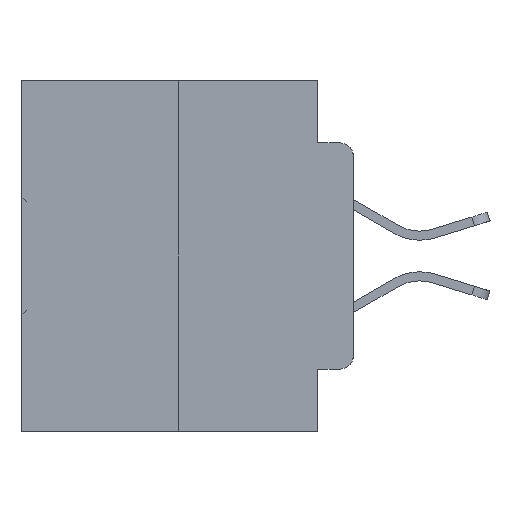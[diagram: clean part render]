
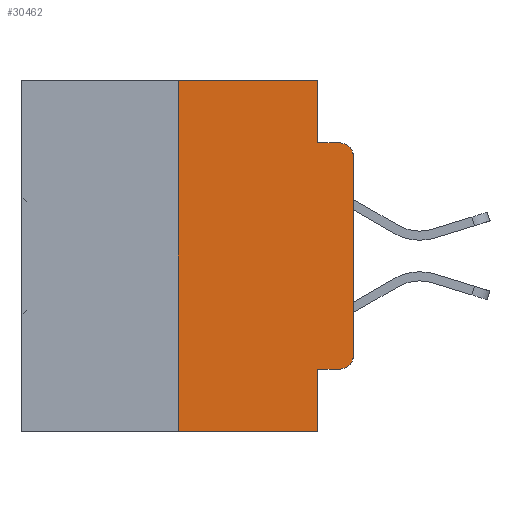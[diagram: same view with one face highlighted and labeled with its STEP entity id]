
A CAD part, left-side view. The second image highlights one B-rep face of the part: STEP entity #30462.
In plain terms, the highlighted planar face has unit normal (-1, 0, 0).
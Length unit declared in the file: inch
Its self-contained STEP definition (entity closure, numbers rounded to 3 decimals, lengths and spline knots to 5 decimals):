
#156 = VERTEX_POINT ( 'NONE', #30643 ) ;
#760 = CARTESIAN_POINT ( 'NONE',  ( 0., 0.02, -0.4115 ) ) ;
#1141 = LINE ( 'NONE', #17078, #32372 ) ;
#1329 = EDGE_CURVE ( 'NONE', #8451, #25424, #10565, .T. ) ;
#2308 = ORIENTED_EDGE ( 'NONE', *, *, #17597, .T. ) ;
#2309 = VERTEX_POINT ( 'NONE', #15167 ) ;
#2852 = LINE ( 'NONE', #10535, #20112 ) ;
#3931 = VERTEX_POINT ( 'NONE', #33849 ) ;
#4574 = EDGE_CURVE ( 'NONE', #19548, #156, #23249, .T. ) ;
#4688 = ORIENTED_EDGE ( 'NONE', *, *, #20201, .T. ) ;
#4934 = DIRECTION ( 'NONE',  ( -1., 0., 0. ) ) ;
#6073 = EDGE_CURVE ( 'NONE', #8706, #3931, #33449, .T. ) ;
#6129 = DIRECTION ( 'NONE',  ( 0., 0., -1. ) ) ;
#6868 = CARTESIAN_POINT ( 'NONE',  ( 0., 0.473, 0. ) ) ;
#7009 = VECTOR ( 'NONE', #31491, 39.37008 ) ;
#8111 = DIRECTION ( 'NONE',  ( 0., 0., 1. ) ) ;
#8451 = VERTEX_POINT ( 'NONE', #20115 ) ;
#8706 = VERTEX_POINT ( 'NONE', #21029 ) ;
#8824 = ORIENTED_EDGE ( 'NONE', *, *, #12725, .T. ) ;
#9120 = EDGE_CURVE ( 'NONE', #19548, #24279, #12750, .T. ) ;
#9899 = LINE ( 'NONE', #20765, #22254 ) ;
#9903 = ORIENTED_EDGE ( 'NONE', *, *, #17345, .F. ) ;
#10204 = CARTESIAN_POINT ( 'NONE',  ( 0., 0.02, -0.3915 ) ) ;
#10334 = CARTESIAN_POINT ( 'NONE',  ( 0., 0.051, -0.4115 ) ) ;
#10535 = CARTESIAN_POINT ( 'NONE',  ( 0., 0.051, -0.0885 ) ) ;
#10545 = LINE ( 'NONE', #23977, #12593 ) ;
#10565 = LINE ( 'NONE', #25010, #22072 ) ;
#11326 = EDGE_CURVE ( 'NONE', #15008, #2309, #1141, .T. ) ;
#12077 = FACE_OUTER_BOUND ( 'NONE', #17263, .T. ) ;
#12593 = VECTOR ( 'NONE', #8111, 39.37008 ) ;
#12725 = EDGE_CURVE ( 'NONE', #24279, #14220, #13362, .T. ) ;
#12750 = LINE ( 'NONE', #10334, #7009 ) ;
#13297 = DIRECTION ( 'NONE',  ( 0., -1., 0. ) ) ;
#13353 = ORIENTED_EDGE ( 'NONE', *, *, #33773, .F. ) ;
#13362 = CIRCLE ( 'NONE', #20995, 0.02 ) ;
#14220 = VERTEX_POINT ( 'NONE', #33222 ) ;
#14357 = CARTESIAN_POINT ( 'NONE',  ( 0., 0.25, 0. ) ) ;
#14895 = VECTOR ( 'NONE', #19980, 39.37008 ) ;
#15008 = VERTEX_POINT ( 'NONE', #23504 ) ;
#15167 = CARTESIAN_POINT ( 'NONE',  ( 0., 0.051, -0.0885 ) ) ;
#16719 = PLANE ( 'NONE',  #16739 ) ;
#16739 = AXIS2_PLACEMENT_3D ( 'NONE', #24525, #24410, #6129 ) ;
#17078 = CARTESIAN_POINT ( 'NONE',  ( 0., 0.051, 0. ) ) ;
#17118 = CARTESIAN_POINT ( 'NONE',  ( 0., 0.02, -0.1085 ) ) ;
#17188 = DIRECTION ( 'NONE',  ( 0., 0., -1. ) ) ;
#17263 = EDGE_LOOP ( 'NONE', ( #4688, #29241, #13353, #27546, #9903, #19221, #2308, #29345, #28546, #8824 ) ) ;
#17345 = EDGE_CURVE ( 'NONE', #25424, #15008, #25975, .T. ) ;
#17519 = CARTESIAN_POINT ( 'NONE',  ( 0., 0.051, 0. ) ) ;
#17597 = EDGE_CURVE ( 'NONE', #8451, #156, #9899, .T. ) ;
#19221 = ORIENTED_EDGE ( 'NONE', *, *, #1329, .F. ) ;
#19548 = VERTEX_POINT ( 'NONE', #29419 ) ;
#19980 = DIRECTION ( 'NONE',  ( 0., -1., 0. ) ) ;
#20112 = VECTOR ( 'NONE', #13297, 39.37008 ) ;
#20115 = CARTESIAN_POINT ( 'NONE',  ( 0., 0.25, -0.5 ) ) ;
#20201 = EDGE_CURVE ( 'NONE', #14220, #8706, #10545, .T. ) ;
#20765 = CARTESIAN_POINT ( 'NONE',  ( 0., 0.473, -0.5 ) ) ;
#20882 = DIRECTION ( 'NONE',  ( 0., -1., 0. ) ) ;
#20995 = AXIS2_PLACEMENT_3D ( 'NONE', #10204, #4934, #28265 ) ;
#21029 = CARTESIAN_POINT ( 'NONE',  ( 0., 0., -0.1085 ) ) ;
#21208 = VECTOR ( 'NONE', #30510, 39.37008 ) ;
#22072 = VECTOR ( 'NONE', #30181, 39.37008 ) ;
#22254 = VECTOR ( 'NONE', #20882, 39.37008 ) ;
#23244 = AXIS2_PLACEMENT_3D ( 'NONE', #17118, #28385, #31008 ) ;
#23249 = LINE ( 'NONE', #17519, #21208 ) ;
#23504 = CARTESIAN_POINT ( 'NONE',  ( 0., 0.051, 0. ) ) ;
#23977 = CARTESIAN_POINT ( 'NONE',  ( 0., 0., 0. ) ) ;
#24279 = VERTEX_POINT ( 'NONE', #760 ) ;
#24410 = DIRECTION ( 'NONE',  ( 1., 0., 0. ) ) ;
#24525 = CARTESIAN_POINT ( 'NONE',  ( 0., 0.473, 0. ) ) ;
#25010 = CARTESIAN_POINT ( 'NONE',  ( 0., 0.25, 0. ) ) ;
#25424 = VERTEX_POINT ( 'NONE', #14357 ) ;
#25975 = LINE ( 'NONE', #6868, #14895 ) ;
#27546 = ORIENTED_EDGE ( 'NONE', *, *, #11326, .F. ) ;
#28265 = DIRECTION ( 'NONE',  ( 0., 0., -1. ) ) ;
#28385 = DIRECTION ( 'NONE',  ( -1., 0., 0. ) ) ;
#28546 = ORIENTED_EDGE ( 'NONE', *, *, #9120, .T. ) ;
#29241 = ORIENTED_EDGE ( 'NONE', *, *, #6073, .T. ) ;
#29345 = ORIENTED_EDGE ( 'NONE', *, *, #4574, .F. ) ;
#29419 = CARTESIAN_POINT ( 'NONE',  ( 0., 0.051, -0.4115 ) ) ;
#30181 = DIRECTION ( 'NONE',  ( 0., 0., 1. ) ) ;
#30462 = ADVANCED_FACE ( 'NONE', ( #12077 ), #16719, .F. ) ;
#30510 = DIRECTION ( 'NONE',  ( 0., 0., -1. ) ) ;
#30643 = CARTESIAN_POINT ( 'NONE',  ( 0., 0.051, -0.5 ) ) ;
#31008 = DIRECTION ( 'NONE',  ( 0., 0., -1. ) ) ;
#31491 = DIRECTION ( 'NONE',  ( 0., -1., 0. ) ) ;
#32372 = VECTOR ( 'NONE', #17188, 39.37008 ) ;
#33222 = CARTESIAN_POINT ( 'NONE',  ( 0., 0., -0.3915 ) ) ;
#33449 = CIRCLE ( 'NONE', #23244, 0.02 ) ;
#33773 = EDGE_CURVE ( 'NONE', #2309, #3931, #2852, .T. ) ;
#33849 = CARTESIAN_POINT ( 'NONE',  ( 0., 0.02, -0.0885 ) ) ;
